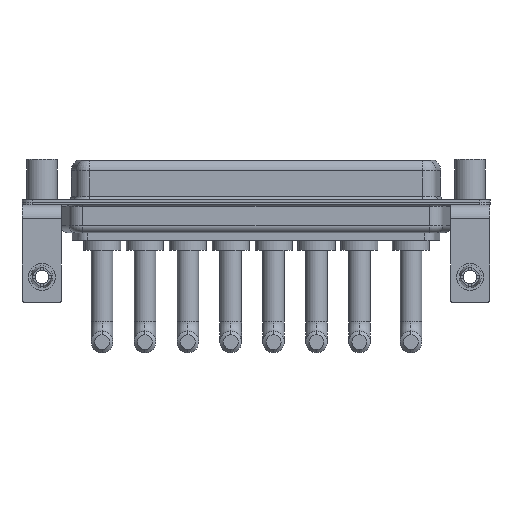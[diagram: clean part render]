
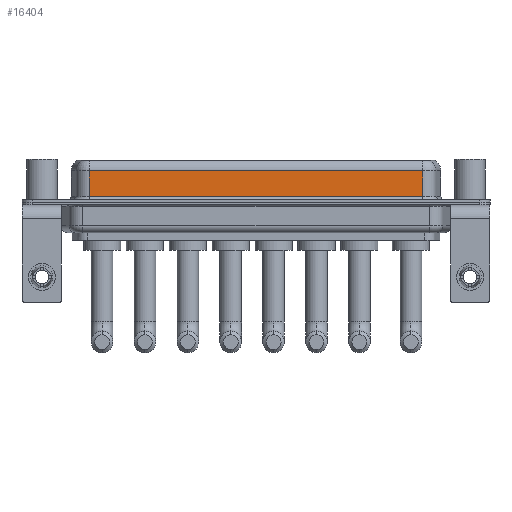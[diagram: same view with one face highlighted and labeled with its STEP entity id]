
A CAD part, front view. The second image highlights one B-rep face of the part: STEP entity #16404.
In plain terms, the highlighted planar face has unit normal (0, -1, 0).
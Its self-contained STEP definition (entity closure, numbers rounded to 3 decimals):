
#14 = CARTESIAN_POINT ( 'NONE',  ( 56.462, -3.95, 0.9 ) ) ;
#362 = ORIENTED_EDGE ( 'NONE', *, *, #9791, .T. ) ;
#943 = ORIENTED_EDGE ( 'NONE', *, *, #2393, .T. ) ;
#1209 = EDGE_LOOP ( 'NONE', ( #8231, #943, #362, #16823 ) ) ;
#2253 = AXIS2_PLACEMENT_3D ( 'NONE', #6344, #6692, #5183 ) ;
#2393 = EDGE_CURVE ( 'NONE', #8330, #14695, #12046, .T. ) ;
#2549 = VERTEX_POINT ( 'NONE', #11882 ) ;
#2728 = CARTESIAN_POINT ( 'NONE',  ( 56.462, -3.95, 6.4 ) ) ;
#2996 = DIRECTION ( 'NONE',  ( 0., 0., -1. ) ) ;
#3285 = VECTOR ( 'NONE', #6777, 1000. ) ;
#3361 = VERTEX_POINT ( 'NONE', #14 ) ;
#3464 = DIRECTION ( 'NONE',  ( 0., 0., -1. ) ) ;
#3748 = CARTESIAN_POINT ( 'NONE',  ( 7.038, -3.95, 4.65 ) ) ;
#3765 = CARTESIAN_POINT ( 'NONE',  ( 56.462, -3.95, 4.65 ) ) ;
#5183 = DIRECTION ( 'NONE',  ( 0., 0., 1. ) ) ;
#6034 = VECTOR ( 'NONE', #10445, 1000. ) ;
#6344 = CARTESIAN_POINT ( 'NONE',  ( 56.462, -3.95, 6.4 ) ) ;
#6692 = DIRECTION ( 'NONE',  ( 0., 1., 0. ) ) ;
#6777 = DIRECTION ( 'NONE',  ( -1., 0., 0. ) ) ;
#8231 = ORIENTED_EDGE ( 'NONE', *, *, #11098, .F. ) ;
#8330 = VERTEX_POINT ( 'NONE', #14979 ) ;
#9511 = LINE ( 'NONE', #2728, #12440 ) ;
#9791 = EDGE_CURVE ( 'NONE', #14695, #2549, #15796, .T. ) ;
#10354 = CARTESIAN_POINT ( 'NONE',  ( 56.462, -3.95, 0.9 ) ) ;
#10445 = DIRECTION ( 'NONE',  ( 1., 0., 0. ) ) ;
#11098 = EDGE_CURVE ( 'NONE', #8330, #3361, #9511, .T. ) ;
#11825 = EDGE_CURVE ( 'NONE', #2549, #3361, #14495, .T. ) ;
#11882 = CARTESIAN_POINT ( 'NONE',  ( 7.038, -3.95, 0.9 ) ) ;
#12046 = LINE ( 'NONE', #3765, #3285 ) ;
#12440 = VECTOR ( 'NONE', #2996, 1000. ) ;
#14440 = PLANE ( 'NONE',  #2253 ) ;
#14495 = LINE ( 'NONE', #10354, #6034 ) ;
#14695 = VERTEX_POINT ( 'NONE', #3748 ) ;
#14979 = CARTESIAN_POINT ( 'NONE',  ( 56.462, -3.95, 4.65 ) ) ;
#15275 = VECTOR ( 'NONE', #3464, 1000. ) ;
#15796 = LINE ( 'NONE', #17187, #15275 ) ;
#16404 = ADVANCED_FACE ( 'NONE', ( #17247 ), #14440, .F. ) ;
#16823 = ORIENTED_EDGE ( 'NONE', *, *, #11825, .T. ) ;
#17187 = CARTESIAN_POINT ( 'NONE',  ( 7.038, -3.95, 6.4 ) ) ;
#17247 = FACE_OUTER_BOUND ( 'NONE', #1209, .T. ) ;
